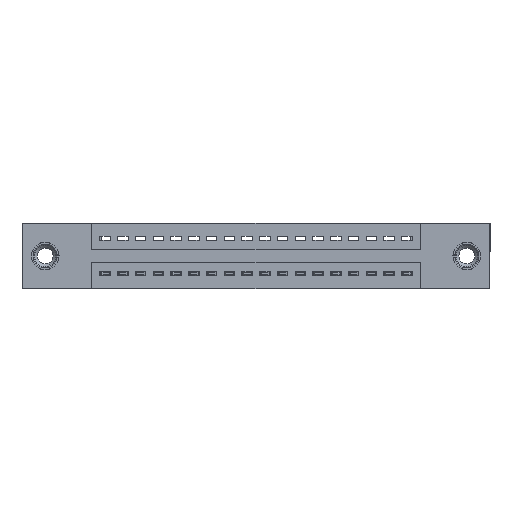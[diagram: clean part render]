
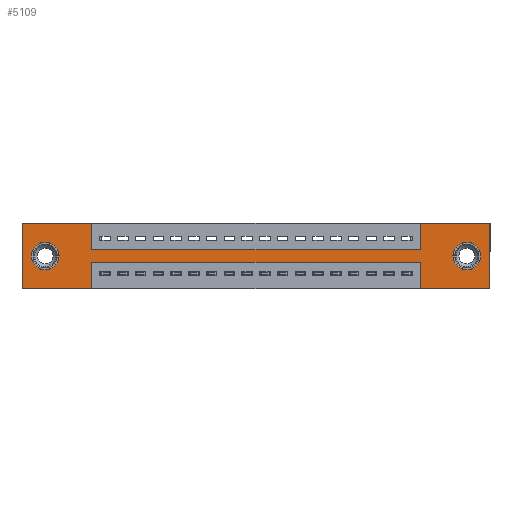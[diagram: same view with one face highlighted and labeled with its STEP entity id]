
A CAD part, front view. The second image highlights one B-rep face of the part: STEP entity #5109.
In plain terms, the highlighted planar face has unit normal (0, -1, 0).
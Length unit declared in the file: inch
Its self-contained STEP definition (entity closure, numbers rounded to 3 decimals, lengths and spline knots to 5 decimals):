
#402 = DIRECTION ( 'NONE',  ( 1., 0., 0. ) ) ;
#647 = LINE ( 'NONE', #8581, #15770 ) ;
#680 = CARTESIAN_POINT ( 'NONE',  ( 2.2425, 0., 0. ) ) ;
#705 = LINE ( 'NONE', #1784, #6770 ) ;
#738 = EDGE_CURVE ( 'NONE', #16951, #14972, #647, .T. ) ;
#852 = VECTOR ( 'NONE', #1331, 39.37008 ) ;
#859 = CARTESIAN_POINT ( 'NONE',  ( 2.2425, 0., -0.37 ) ) ;
#1001 = CARTESIAN_POINT ( 'NONE',  ( 0., 0., 0. ) ) ;
#1063 = CARTESIAN_POINT ( 'NONE',  ( 2.505, 0., -0.263 ) ) ;
#1073 = DIRECTION ( 'NONE',  ( 1., 0., 0. ) ) ;
#1093 = CARTESIAN_POINT ( 'NONE',  ( 0., 0., 0. ) ) ;
#1331 = DIRECTION ( 'NONE',  ( -1., 0., 0. ) ) ;
#1333 = CIRCLE ( 'NONE', #4114, 0.078 ) ;
#1526 = LINE ( 'NONE', #680, #10965 ) ;
#1764 = ORIENTED_EDGE ( 'NONE', *, *, #10930, .F. ) ;
#1767 = CARTESIAN_POINT ( 'NONE',  ( 0.3925, 0., -0.37 ) ) ;
#1784 = CARTESIAN_POINT ( 'NONE',  ( 0., 0., 0. ) ) ;
#1886 = ORIENTED_EDGE ( 'NONE', *, *, #7256, .F. ) ;
#2158 = DIRECTION ( 'NONE',  ( 0., -1., 0. ) ) ;
#2606 = CARTESIAN_POINT ( 'NONE',  ( 0., 0., -0.37 ) ) ;
#2644 = LINE ( 'NONE', #12749, #6692 ) ;
#2949 = CARTESIAN_POINT ( 'NONE',  ( 2.2425, 0., -0.22 ) ) ;
#3042 = DIRECTION ( 'NONE',  ( 0., 1., 0. ) ) ;
#3352 = VERTEX_POINT ( 'NONE', #6803 ) ;
#3610 = LINE ( 'NONE', #5648, #6519 ) ;
#3628 = VECTOR ( 'NONE', #402, 39.37008 ) ;
#3644 = ORIENTED_EDGE ( 'NONE', *, *, #17919, .T. ) ;
#3805 = VERTEX_POINT ( 'NONE', #13275 ) ;
#3885 = AXIS2_PLACEMENT_3D ( 'NONE', #5897, #3042, #4783 ) ;
#3901 = LINE ( 'NONE', #1093, #13150 ) ;
#3930 = EDGE_CURVE ( 'NONE', #18460, #18757, #1333, .T. ) ;
#4001 = DIRECTION ( 'NONE',  ( -1., 0., 0. ) ) ;
#4081 = DIRECTION ( 'NONE',  ( 0., 0., -1. ) ) ;
#4114 = AXIS2_PLACEMENT_3D ( 'NONE', #12523, #5458, #6777 ) ;
#4267 = CARTESIAN_POINT ( 'NONE',  ( 0.13, 0., -0.263 ) ) ;
#4398 = CARTESIAN_POINT ( 'NONE',  ( 2.505, 0., -0.185 ) ) ;
#4476 = VECTOR ( 'NONE', #8639, 39.37008 ) ;
#4499 = ORIENTED_EDGE ( 'NONE', *, *, #5839, .F. ) ;
#4548 = VERTEX_POINT ( 'NONE', #2606 ) ;
#4581 = DIRECTION ( 'NONE',  ( 0., 1., 0. ) ) ;
#4673 = VECTOR ( 'NONE', #16511, 39.37008 ) ;
#4783 = DIRECTION ( 'NONE',  ( 0., 0., 1. ) ) ;
#5109 = ADVANCED_FACE ( 'NONE', ( #12261, #13610, #13398 ), #9528, .T. ) ;
#5220 = DIRECTION ( 'NONE',  ( 0., 0., 1. ) ) ;
#5458 = DIRECTION ( 'NONE',  ( 0., 1., 0. ) ) ;
#5560 = AXIS2_PLACEMENT_3D ( 'NONE', #13791, #2158, #8004 ) ;
#5648 = CARTESIAN_POINT ( 'NONE',  ( 0., 0., 0. ) ) ;
#5825 = VECTOR ( 'NONE', #4081, 39.37008 ) ;
#5839 = EDGE_CURVE ( 'NONE', #4548, #18257, #3901, .T. ) ;
#5897 = CARTESIAN_POINT ( 'NONE',  ( 0.13, 0., -0.185 ) ) ;
#6239 = ORIENTED_EDGE ( 'NONE', *, *, #18502, .F. ) ;
#6519 = VECTOR ( 'NONE', #1073, 39.37008 ) ;
#6576 = CARTESIAN_POINT ( 'NONE',  ( 2.635, 0., 0. ) ) ;
#6692 = VECTOR ( 'NONE', #4001, 39.37008 ) ;
#6770 = VECTOR ( 'NONE', #8952, 39.37008 ) ;
#6777 = DIRECTION ( 'NONE',  ( 0., 0., -1. ) ) ;
#6803 = CARTESIAN_POINT ( 'NONE',  ( 2.635, 0., 0. ) ) ;
#6819 = CARTESIAN_POINT ( 'NONE',  ( 2.2425, 0., -0.15 ) ) ;
#7256 = EDGE_CURVE ( 'NONE', #12283, #13575, #11511, .T. ) ;
#7282 = CARTESIAN_POINT ( 'NONE',  ( 0.3925, 0., -0.22 ) ) ;
#7356 = CARTESIAN_POINT ( 'NONE',  ( 0.3925, 0., 0. ) ) ;
#7408 = LINE ( 'NONE', #10150, #4476 ) ;
#7578 = CARTESIAN_POINT ( 'NONE',  ( 2.505, 0., -0.107 ) ) ;
#7623 = EDGE_CURVE ( 'NONE', #15947, #3352, #3610, .T. ) ;
#7629 = CIRCLE ( 'NONE', #12350, 0.078 ) ;
#7660 = VERTEX_POINT ( 'NONE', #10746 ) ;
#7662 = DIRECTION ( 'NONE',  ( 0., 0., 1. ) ) ;
#7725 = CARTESIAN_POINT ( 'NONE',  ( 0.13, 0., -0.185 ) ) ;
#7818 = ORIENTED_EDGE ( 'NONE', *, *, #18001, .F. ) ;
#8004 = DIRECTION ( 'NONE',  ( 0., 0., -1. ) ) ;
#8148 = ORIENTED_EDGE ( 'NONE', *, *, #3930, .T. ) ;
#8154 = ORIENTED_EDGE ( 'NONE', *, *, #738, .F. ) ;
#8581 = CARTESIAN_POINT ( 'NONE',  ( 2.2425, 0., -0.37 ) ) ;
#8639 = DIRECTION ( 'NONE',  ( 0., 0., -1. ) ) ;
#8660 = ORIENTED_EDGE ( 'NONE', *, *, #7623, .F. ) ;
#8862 = EDGE_CURVE ( 'NONE', #3805, #18554, #7629, .T. ) ;
#8952 = DIRECTION ( 'NONE',  ( 1., 0., 0. ) ) ;
#9528 = PLANE ( 'NONE',  #5560 ) ;
#9989 = EDGE_CURVE ( 'NONE', #3352, #17692, #18057, .T. ) ;
#10033 = VERTEX_POINT ( 'NONE', #17698 ) ;
#10150 = CARTESIAN_POINT ( 'NONE',  ( 0.3925, 0., -0.37 ) ) ;
#10480 = EDGE_CURVE ( 'NONE', #17692, #16951, #13683, .T. ) ;
#10557 = EDGE_CURVE ( 'NONE', #15169, #4548, #2644, .T. ) ;
#10746 = CARTESIAN_POINT ( 'NONE',  ( 0.3925, 0., 0. ) ) ;
#10857 = CARTESIAN_POINT ( 'NONE',  ( 0., 0., -0.37 ) ) ;
#10903 = ORIENTED_EDGE ( 'NONE', *, *, #17259, .T. ) ;
#10930 = EDGE_CURVE ( 'NONE', #13575, #15947, #1526, .T. ) ;
#10965 = VECTOR ( 'NONE', #16571, 39.37008 ) ;
#10986 = EDGE_LOOP ( 'NONE', ( #3644, #8148 ) ) ;
#11076 = CARTESIAN_POINT ( 'NONE',  ( 2.635, 0., -0.37 ) ) ;
#11236 = CIRCLE ( 'NONE', #17709, 0.078 ) ;
#11290 = CARTESIAN_POINT ( 'NONE',  ( 0.3925, 0., -0.15 ) ) ;
#11349 = ORIENTED_EDGE ( 'NONE', *, *, #10480, .F. ) ;
#11458 = LINE ( 'NONE', #7356, #12359 ) ;
#11511 = LINE ( 'NONE', #17954, #3628 ) ;
#11763 = DIRECTION ( 'NONE',  ( 0., 0., -1. ) ) ;
#11923 = CARTESIAN_POINT ( 'NONE',  ( 2.2425, 0., 0. ) ) ;
#12261 = FACE_BOUND ( 'NONE', #10986, .T. ) ;
#12283 = VERTEX_POINT ( 'NONE', #11290 ) ;
#12350 = AXIS2_PLACEMENT_3D ( 'NONE', #7725, #4581, #7662 ) ;
#12359 = VECTOR ( 'NONE', #11763, 39.37008 ) ;
#12472 = DIRECTION ( 'NONE',  ( 0., 0., 1. ) ) ;
#12523 = CARTESIAN_POINT ( 'NONE',  ( 2.505, 0., -0.185 ) ) ;
#12749 = CARTESIAN_POINT ( 'NONE',  ( 0., 0., -0.37 ) ) ;
#13149 = DIRECTION ( 'NONE',  ( 0., 0., -1. ) ) ;
#13150 = VECTOR ( 'NONE', #5220, 39.37008 ) ;
#13264 = DIRECTION ( 'NONE',  ( 0., 1., 0. ) ) ;
#13275 = CARTESIAN_POINT ( 'NONE',  ( 0.13, 0., -0.107 ) ) ;
#13398 = FACE_OUTER_BOUND ( 'NONE', #16359, .T. ) ;
#13575 = VERTEX_POINT ( 'NONE', #6819 ) ;
#13594 = ORIENTED_EDGE ( 'NONE', *, *, #14194, .F. ) ;
#13610 = FACE_BOUND ( 'NONE', #14414, .T. ) ;
#13683 = LINE ( 'NONE', #10857, #4673 ) ;
#13791 = CARTESIAN_POINT ( 'NONE',  ( 0., 0., -0.37 ) ) ;
#14194 = EDGE_CURVE ( 'NONE', #18257, #7660, #705, .T. ) ;
#14414 = EDGE_LOOP ( 'NONE', ( #18733, #10903 ) ) ;
#14972 = VERTEX_POINT ( 'NONE', #2949 ) ;
#15169 = VERTEX_POINT ( 'NONE', #1767 ) ;
#15451 = ORIENTED_EDGE ( 'NONE', *, *, #9989, .F. ) ;
#15770 = VECTOR ( 'NONE', #12472, 39.37008 ) ;
#15947 = VERTEX_POINT ( 'NONE', #11923 ) ;
#16359 = EDGE_LOOP ( 'NONE', ( #18212, #6239, #8154, #11349, #15451, #8660, #1764, #1886, #7818, #13594, #4499, #17640 ) ) ;
#16480 = CIRCLE ( 'NONE', #3885, 0.078 ) ;
#16511 = DIRECTION ( 'NONE',  ( -1., 0., 0. ) ) ;
#16571 = DIRECTION ( 'NONE',  ( 0., 0., 1. ) ) ;
#16655 = LINE ( 'NONE', #7282, #852 ) ;
#16951 = VERTEX_POINT ( 'NONE', #859 ) ;
#17259 = EDGE_CURVE ( 'NONE', #18554, #3805, #16480, .T. ) ;
#17640 = ORIENTED_EDGE ( 'NONE', *, *, #10557, .F. ) ;
#17692 = VERTEX_POINT ( 'NONE', #11076 ) ;
#17698 = CARTESIAN_POINT ( 'NONE',  ( 0.3925, 0., -0.22 ) ) ;
#17709 = AXIS2_PLACEMENT_3D ( 'NONE', #4398, #13264, #13149 ) ;
#17859 = EDGE_CURVE ( 'NONE', #10033, #15169, #7408, .T. ) ;
#17919 = EDGE_CURVE ( 'NONE', #18757, #18460, #11236, .T. ) ;
#17954 = CARTESIAN_POINT ( 'NONE',  ( 0.3925, 0., -0.15 ) ) ;
#18001 = EDGE_CURVE ( 'NONE', #7660, #12283, #11458, .T. ) ;
#18057 = LINE ( 'NONE', #6576, #5825 ) ;
#18212 = ORIENTED_EDGE ( 'NONE', *, *, #17859, .F. ) ;
#18257 = VERTEX_POINT ( 'NONE', #1001 ) ;
#18460 = VERTEX_POINT ( 'NONE', #1063 ) ;
#18502 = EDGE_CURVE ( 'NONE', #14972, #10033, #16655, .T. ) ;
#18554 = VERTEX_POINT ( 'NONE', #4267 ) ;
#18733 = ORIENTED_EDGE ( 'NONE', *, *, #8862, .T. ) ;
#18757 = VERTEX_POINT ( 'NONE', #7578 ) ;
